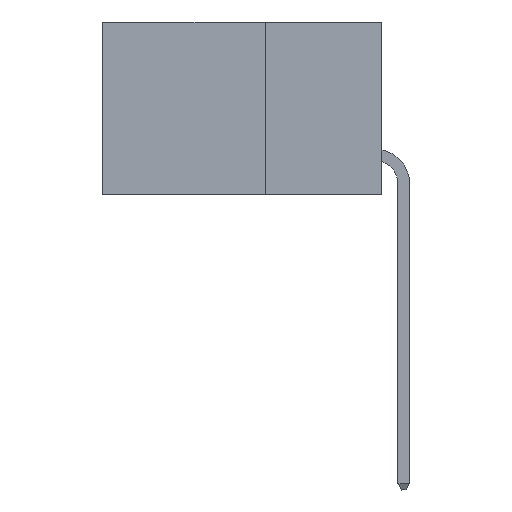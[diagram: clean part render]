
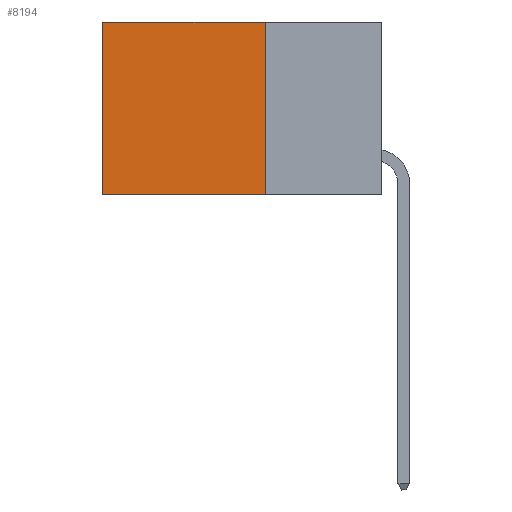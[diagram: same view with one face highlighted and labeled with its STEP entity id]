
A CAD part, left-side view. The second image highlights one B-rep face of the part: STEP entity #8194.
In plain terms, the highlighted planar face has unit normal (-1, 0, 0).
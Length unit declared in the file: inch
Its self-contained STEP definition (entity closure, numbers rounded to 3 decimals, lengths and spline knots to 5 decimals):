
#1695 = CARTESIAN_POINT ( 'NONE',  ( 0.2875, 0.6, -0.37 ) ) ;
#2915 = VECTOR ( 'NONE', #28683, 39.37008 ) ;
#3669 = EDGE_CURVE ( 'NONE', #35218, #37692, #29614, .T. ) ;
#3905 = FACE_OUTER_BOUND ( 'NONE', #5180, .T. ) ;
#4277 = LINE ( 'NONE', #4847, #2915 ) ;
#4847 = CARTESIAN_POINT ( 'NONE',  ( 0.2875, 0.25, 0. ) ) ;
#5180 = EDGE_LOOP ( 'NONE', ( #19654, #33214, #26228, #28659 ) ) ;
#7511 = DIRECTION ( 'NONE',  ( 0., 0., -1. ) ) ;
#7519 = LINE ( 'NONE', #25996, #14517 ) ;
#8194 = ADVANCED_FACE ( 'NONE', ( #3905 ), #29594, .F. ) ;
#11268 = LINE ( 'NONE', #16179, #26067 ) ;
#12814 = CARTESIAN_POINT ( 'NONE',  ( 0.2875, 0.6, 0. ) ) ;
#13081 = EDGE_CURVE ( 'NONE', #35218, #33783, #4277, .T. ) ;
#13430 = VECTOR ( 'NONE', #7511, 39.37008 ) ;
#14517 = VECTOR ( 'NONE', #34704, 39.37008 ) ;
#16179 = CARTESIAN_POINT ( 'NONE',  ( 0.2875, 0.6, 0. ) ) ;
#17359 = DIRECTION ( 'NONE',  ( 0., 0., -1. ) ) ;
#18977 = AXIS2_PLACEMENT_3D ( 'NONE', #32207, #26207, #17359 ) ;
#19189 = CARTESIAN_POINT ( 'NONE',  ( 0.2875, 0.25, -0.37 ) ) ;
#19566 = CARTESIAN_POINT ( 'NONE',  ( 0.2875, 0.25, 0. ) ) ;
#19648 = DIRECTION ( 'NONE',  ( 0., 0., -1. ) ) ;
#19654 = ORIENTED_EDGE ( 'NONE', *, *, #20019, .T. ) ;
#20019 = EDGE_CURVE ( 'NONE', #33783, #25309, #11268, .T. ) ;
#25309 = VERTEX_POINT ( 'NONE', #1695 ) ;
#25996 = CARTESIAN_POINT ( 'NONE',  ( 0.2875, 0.25, -0.37 ) ) ;
#26067 = VECTOR ( 'NONE', #19648, 39.37008 ) ;
#26207 = DIRECTION ( 'NONE',  ( 1., 0., 0. ) ) ;
#26228 = ORIENTED_EDGE ( 'NONE', *, *, #3669, .F. ) ;
#28659 = ORIENTED_EDGE ( 'NONE', *, *, #13081, .T. ) ;
#28683 = DIRECTION ( 'NONE',  ( 0., 1., 0. ) ) ;
#29594 = PLANE ( 'NONE',  #18977 ) ;
#29614 = LINE ( 'NONE', #19566, #13430 ) ;
#32207 = CARTESIAN_POINT ( 'NONE',  ( 0.2875, 0.25, 0. ) ) ;
#33214 = ORIENTED_EDGE ( 'NONE', *, *, #37867, .F. ) ;
#33783 = VERTEX_POINT ( 'NONE', #12814 ) ;
#34704 = DIRECTION ( 'NONE',  ( 0., 1., 0. ) ) ;
#35218 = VERTEX_POINT ( 'NONE', #37044 ) ;
#37044 = CARTESIAN_POINT ( 'NONE',  ( 0.2875, 0.25, 0. ) ) ;
#37692 = VERTEX_POINT ( 'NONE', #19189 ) ;
#37867 = EDGE_CURVE ( 'NONE', #37692, #25309, #7519, .T. ) ;
